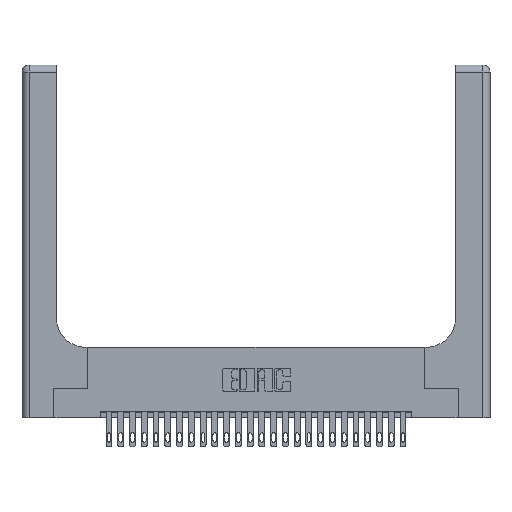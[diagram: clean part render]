
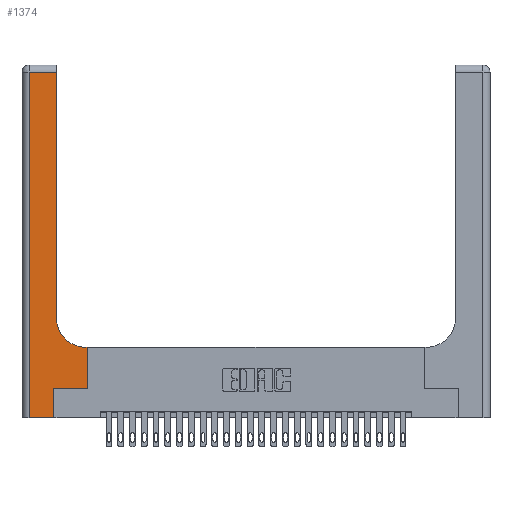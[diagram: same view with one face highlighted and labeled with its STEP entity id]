
A CAD part, top view. The second image highlights one B-rep face of the part: STEP entity #1374.
In plain terms, the highlighted planar face has unit normal (0, 0, 1).
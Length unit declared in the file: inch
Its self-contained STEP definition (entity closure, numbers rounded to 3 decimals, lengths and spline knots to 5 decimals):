
#361 = EDGE_CURVE ( 'NONE', #24217, #19584, #6473, .T. ) ;
#516 = DIRECTION ( 'NONE',  ( 1., 0., 0. ) ) ;
#798 = CARTESIAN_POINT ( 'NONE',  ( 0.5585, 0.25, 0.37 ) ) ;
#1125 = EDGE_CURVE ( 'NONE', #17455, #26197, #18128, .T. ) ;
#1374 = ADVANCED_FACE ( 'NONE', ( #15093 ), #19868, .F. ) ;
#1769 = CARTESIAN_POINT ( 'NONE',  ( 0.269, 0., 0.37 ) ) ;
#2164 = DIRECTION ( 'NONE',  ( 1., 0., 0. ) ) ;
#2517 = DIRECTION ( 'NONE',  ( 0., 0., -1. ) ) ;
#2542 = VERTEX_POINT ( 'NONE', #10450 ) ;
#2724 = ORIENTED_EDGE ( 'NONE', *, *, #25649, .T. ) ;
#2879 = CARTESIAN_POINT ( 'NONE',  ( 0., 3., 0.37 ) ) ;
#3086 = EDGE_CURVE ( 'NONE', #10020, #17455, #16378, .T. ) ;
#3152 = DIRECTION ( 'NONE',  ( 0., 1., 0. ) ) ;
#3366 = LINE ( 'NONE', #27632, #23382 ) ;
#4138 = DIRECTION ( 'NONE',  ( 0., 1., 0. ) ) ;
#5378 = EDGE_CURVE ( 'NONE', #19584, #11770, #9544, .T. ) ;
#6473 = LINE ( 'NONE', #19537, #20132 ) ;
#6682 = EDGE_CURVE ( 'NONE', #25842, #23406, #22831, .T. ) ;
#7085 = DIRECTION ( 'NONE',  ( 0., -1., 0. ) ) ;
#7212 = AXIS2_PLACEMENT_3D ( 'NONE', #12896, #2517, #516 ) ;
#8250 = ORIENTED_EDGE ( 'NONE', *, *, #24117, .T. ) ;
#8423 = EDGE_CURVE ( 'NONE', #26197, #24217, #26412, .T. ) ;
#8692 = CARTESIAN_POINT ( 'NONE',  ( 0.2915, 2.94, 0.37 ) ) ;
#8745 = ORIENTED_EDGE ( 'NONE', *, *, #15507, .T. ) ;
#8945 = DIRECTION ( 'NONE',  ( 0., 1., 0. ) ) ;
#9544 = LINE ( 'NONE', #12895, #21240 ) ;
#10020 = VERTEX_POINT ( 'NONE', #18946 ) ;
#10450 = CARTESIAN_POINT ( 'NONE',  ( 0.5585, 0.25, 0.37 ) ) ;
#10680 = LINE ( 'NONE', #798, #23684 ) ;
#10789 = ORIENTED_EDGE ( 'NONE', *, *, #3086, .T. ) ;
#11484 = VECTOR ( 'NONE', #4138, 39.37008 ) ;
#11770 = VERTEX_POINT ( 'NONE', #12114 ) ;
#11922 = CARTESIAN_POINT ( 'NONE',  ( 0.2915, 0.6, 0.37 ) ) ;
#12114 = CARTESIAN_POINT ( 'NONE',  ( 0.06, 0., 0.37 ) ) ;
#12486 = CARTESIAN_POINT ( 'NONE',  ( 0.269, 0.25, 0.37 ) ) ;
#12567 = DIRECTION ( 'NONE',  ( -1., 0., 0. ) ) ;
#12895 = CARTESIAN_POINT ( 'NONE',  ( 0.06, 3., 0.37 ) ) ;
#12896 = CARTESIAN_POINT ( 'NONE',  ( 0.5415, 0.85, 0.37 ) ) ;
#12929 = ORIENTED_EDGE ( 'NONE', *, *, #8423, .T. ) ;
#13074 = DIRECTION ( 'NONE',  ( -1., 0., 0. ) ) ;
#13342 = VECTOR ( 'NONE', #12567, 39.37008 ) ;
#14066 = DIRECTION ( 'NONE',  ( 1., 0., 0. ) ) ;
#15093 = FACE_OUTER_BOUND ( 'NONE', #17592, .T. ) ;
#15507 = EDGE_CURVE ( 'NONE', #11770, #25842, #16526, .T. ) ;
#15785 = CARTESIAN_POINT ( 'NONE',  ( 0.5415, 0.6, 0.37 ) ) ;
#15838 = ORIENTED_EDGE ( 'NONE', *, *, #6682, .T. ) ;
#16378 = LINE ( 'NONE', #11922, #13342 ) ;
#16526 = LINE ( 'NONE', #22719, #24474 ) ;
#17455 = VERTEX_POINT ( 'NONE', #15785 ) ;
#17592 = EDGE_LOOP ( 'NONE', ( #12929, #24259, #25850, #8745, #15838, #8250, #2724, #10789, #25099 ) ) ;
#17777 = AXIS2_PLACEMENT_3D ( 'NONE', #2879, #18203, #24515 ) ;
#18128 = CIRCLE ( 'NONE', #7212, 0.25 ) ;
#18203 = DIRECTION ( 'NONE',  ( 0., 0., -1. ) ) ;
#18384 = CARTESIAN_POINT ( 'NONE',  ( 0.269, 0., 0.37 ) ) ;
#18946 = CARTESIAN_POINT ( 'NONE',  ( 0.5585, 0.6, 0.37 ) ) ;
#19505 = CARTESIAN_POINT ( 'NONE',  ( 0.2915, 3., 0.37 ) ) ;
#19537 = CARTESIAN_POINT ( 'NONE',  ( 0., 2.94, 0.37 ) ) ;
#19584 = VERTEX_POINT ( 'NONE', #23803 ) ;
#19868 = PLANE ( 'NONE',  #17777 ) ;
#20132 = VECTOR ( 'NONE', #13074, 39.37008 ) ;
#21240 = VECTOR ( 'NONE', #7085, 39.37008 ) ;
#22719 = CARTESIAN_POINT ( 'NONE',  ( 0., 0., 0.37 ) ) ;
#22831 = LINE ( 'NONE', #1769, #11484 ) ;
#23382 = VECTOR ( 'NONE', #2164, 39.37008 ) ;
#23406 = VERTEX_POINT ( 'NONE', #12486 ) ;
#23684 = VECTOR ( 'NONE', #3152, 39.37008 ) ;
#23803 = CARTESIAN_POINT ( 'NONE',  ( 0.06, 2.94, 0.37 ) ) ;
#24117 = EDGE_CURVE ( 'NONE', #23406, #2542, #3366, .T. ) ;
#24217 = VERTEX_POINT ( 'NONE', #8692 ) ;
#24259 = ORIENTED_EDGE ( 'NONE', *, *, #361, .T. ) ;
#24474 = VECTOR ( 'NONE', #14066, 39.37008 ) ;
#24515 = DIRECTION ( 'NONE',  ( -1., 0., 0. ) ) ;
#24748 = VECTOR ( 'NONE', #8945, 39.37008 ) ;
#25099 = ORIENTED_EDGE ( 'NONE', *, *, #1125, .T. ) ;
#25649 = EDGE_CURVE ( 'NONE', #2542, #10020, #10680, .T. ) ;
#25842 = VERTEX_POINT ( 'NONE', #18384 ) ;
#25850 = ORIENTED_EDGE ( 'NONE', *, *, #5378, .T. ) ;
#26197 = VERTEX_POINT ( 'NONE', #26462 ) ;
#26412 = LINE ( 'NONE', #19505, #24748 ) ;
#26462 = CARTESIAN_POINT ( 'NONE',  ( 0.2915, 0.85, 0.37 ) ) ;
#27632 = CARTESIAN_POINT ( 'NONE',  ( 0.269, 0.25, 0.37 ) ) ;
